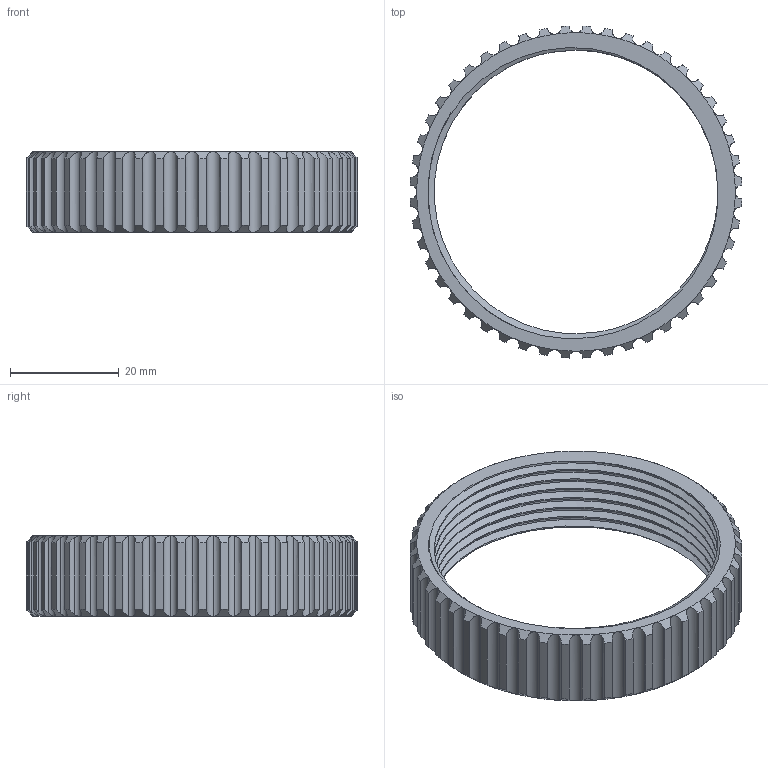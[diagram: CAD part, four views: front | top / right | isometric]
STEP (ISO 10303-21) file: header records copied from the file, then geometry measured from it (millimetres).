
FILE_DESCRIPTION (( 'STEP AP203' ), '1' );
FILE_NAME ('AF-22LRPP-SB-PRT-003-STEP.STEP', '2020-08-30T11:15:57', ( '' ), ( '' ), 'SwSTEP 2.0', 'SolidWorks 2018', '' );
FILE_SCHEMA (( 'CONFIG_CONTROL_DESIGN' ));
Length unit declared in the file: inch
Products named in the file (1): AF-22LRPP-SB-PRT-003-STEP
Bounding box: 60.91 x 60.91 x 14.82 mm (x, y, z)
Volume: 8192.5 mm3; surface area: 8731 mm2
Topology: 1 solids, 1 shells, 235 faces, 601 edges, 368 vertices
Faces by surface type: cylinder 134, cone 96, bspline 3, plane 2
Entity records: 10597 total; most frequent: CARTESIAN_POINT 5286, ORIENTED_EDGE 1202, DIRECTION 987, EDGE_CURVE 601, AXIS2_PLACEMENT_3D 427, VERTEX_POINT 368, B_SPLINE_CURVE_WITH_KNOTS 242, EDGE_LOOP 237
